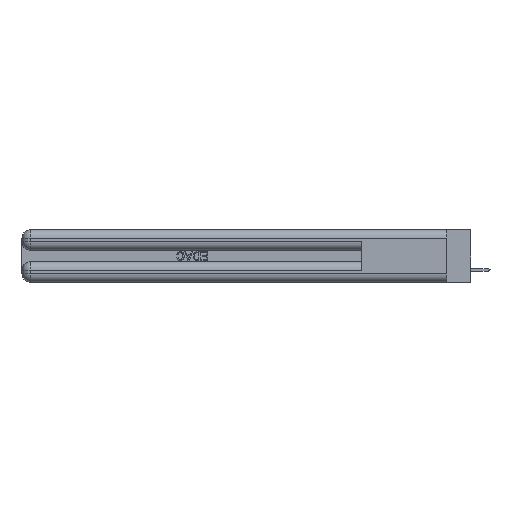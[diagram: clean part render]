
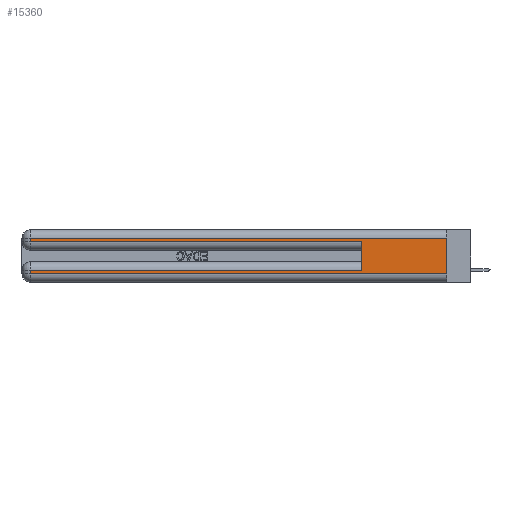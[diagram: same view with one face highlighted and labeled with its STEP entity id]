
A CAD part, left-side view. The second image highlights one B-rep face of the part: STEP entity #15360.
In plain terms, the highlighted planar face has unit normal (-1, 0, 0).
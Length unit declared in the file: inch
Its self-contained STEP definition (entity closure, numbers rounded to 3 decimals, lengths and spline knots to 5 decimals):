
#1582 = CARTESIAN_POINT ( 'NONE',  ( 0., 0.6, 0.285 ) ) ;
#2096 = CARTESIAN_POINT ( 'NONE',  ( 0., 2.94, 0.37 ) ) ;
#4617 = DIRECTION ( 'NONE',  ( 0., 1., 0. ) ) ;
#4679 = LINE ( 'NONE', #52619, #6367 ) ;
#5999 = ORIENTED_EDGE ( 'NONE', *, *, #34474, .T. ) ;
#6293 = VECTOR ( 'NONE', #22953, 39.37008 ) ;
#6367 = VECTOR ( 'NONE', #24795, 39.37008 ) ;
#7315 = LINE ( 'NONE', #24881, #41781 ) ;
#9867 = EDGE_CURVE ( 'NONE', #53524, #52220, #13985, .T. ) ;
#9911 = VERTEX_POINT ( 'NONE', #38701 ) ;
#11343 = ORIENTED_EDGE ( 'NONE', *, *, #21240, .T. ) ;
#13246 = ORIENTED_EDGE ( 'NONE', *, *, #28606, .F. ) ;
#13438 = FACE_OUTER_BOUND ( 'NONE', #19510, .T. ) ;
#13985 = LINE ( 'NONE', #18338, #6293 ) ;
#14717 = CARTESIAN_POINT ( 'NONE',  ( 0., 0., 0.37 ) ) ;
#14865 = VECTOR ( 'NONE', #4617, 39.37008 ) ;
#15360 = ADVANCED_FACE ( 'NONE', ( #13438 ), #34341, .F. ) ;
#17070 = ORIENTED_EDGE ( 'NONE', *, *, #25640, .T. ) ;
#17555 = ORIENTED_EDGE ( 'NONE', *, *, #9867, .T. ) ;
#17757 = CARTESIAN_POINT ( 'NONE',  ( 0., 2.94, 0.06 ) ) ;
#17925 = CARTESIAN_POINT ( 'NONE',  ( 0., 0., 0.31 ) ) ;
#18238 = VERTEX_POINT ( 'NONE', #35197 ) ;
#18338 = CARTESIAN_POINT ( 'NONE',  ( 0., 2.94, 0.37 ) ) ;
#19503 = CARTESIAN_POINT ( 'NONE',  ( 0., 2.94, 0.31 ) ) ;
#19510 = EDGE_LOOP ( 'NONE', ( #13246, #17070, #52996, #36879, #20248, #11343, #17555, #5999 ) ) ;
#20248 = ORIENTED_EDGE ( 'NONE', *, *, #52479, .F. ) ;
#21240 = EDGE_CURVE ( 'NONE', #18238, #53524, #4679, .T. ) ;
#22718 = LINE ( 'NONE', #2096, #28670 ) ;
#22953 = DIRECTION ( 'NONE',  ( 0., 0., -1. ) ) ;
#23076 = CARTESIAN_POINT ( 'NONE',  ( 0., 0., 0.06 ) ) ;
#24795 = DIRECTION ( 'NONE',  ( 0., 1., 0. ) ) ;
#24881 = CARTESIAN_POINT ( 'NONE',  ( 0., 0., 0.37 ) ) ;
#25640 = EDGE_CURVE ( 'NONE', #30573, #50424, #33668, .T. ) ;
#27232 = VERTEX_POINT ( 'NONE', #1582 ) ;
#27782 = DIRECTION ( 'NONE',  ( 0., 0., 1. ) ) ;
#27937 = LINE ( 'NONE', #23076, #38654 ) ;
#28046 = LINE ( 'NONE', #28839, #50780 ) ;
#28440 = CARTESIAN_POINT ( 'NONE',  ( 0., 2.94, 0.085 ) ) ;
#28606 = EDGE_CURVE ( 'NONE', #30573, #9911, #7315, .T. ) ;
#28670 = VECTOR ( 'NONE', #51251, 39.37008 ) ;
#28839 = CARTESIAN_POINT ( 'NONE',  ( 0., 0.6, 0.145 ) ) ;
#29768 = VECTOR ( 'NONE', #53421, 39.37008 ) ;
#30091 = EDGE_CURVE ( 'NONE', #37334, #27232, #32470, .T. ) ;
#30394 = CARTESIAN_POINT ( 'NONE',  ( 0., 0., 0.31 ) ) ;
#30573 = VERTEX_POINT ( 'NONE', #17925 ) ;
#32470 = LINE ( 'NONE', #41150, #29768 ) ;
#32953 = AXIS2_PLACEMENT_3D ( 'NONE', #14717, #38137, #48127 ) ;
#33668 = LINE ( 'NONE', #30394, #14865 ) ;
#34341 = PLANE ( 'NONE',  #32953 ) ;
#34474 = EDGE_CURVE ( 'NONE', #52220, #9911, #27937, .T. ) ;
#35197 = CARTESIAN_POINT ( 'NONE',  ( 0., 0.6, 0.085 ) ) ;
#36879 = ORIENTED_EDGE ( 'NONE', *, *, #30091, .T. ) ;
#37334 = VERTEX_POINT ( 'NONE', #41822 ) ;
#38137 = DIRECTION ( 'NONE',  ( 1., 0., 0. ) ) ;
#38654 = VECTOR ( 'NONE', #39628, 39.37008 ) ;
#38701 = CARTESIAN_POINT ( 'NONE',  ( 0., 0., 0.06 ) ) ;
#39628 = DIRECTION ( 'NONE',  ( 0., -1., 0. ) ) ;
#40443 = DIRECTION ( 'NONE',  ( 0., 0., -1. ) ) ;
#41150 = CARTESIAN_POINT ( 'NONE',  ( 0., 0., 0.285 ) ) ;
#41781 = VECTOR ( 'NONE', #40443, 39.37008 ) ;
#41822 = CARTESIAN_POINT ( 'NONE',  ( 0., 2.94, 0.285 ) ) ;
#45332 = EDGE_CURVE ( 'NONE', #50424, #37334, #22718, .T. ) ;
#48127 = DIRECTION ( 'NONE',  ( 0., 0., -1. ) ) ;
#50424 = VERTEX_POINT ( 'NONE', #19503 ) ;
#50780 = VECTOR ( 'NONE', #27782, 39.37008 ) ;
#51251 = DIRECTION ( 'NONE',  ( 0., 0., -1. ) ) ;
#52220 = VERTEX_POINT ( 'NONE', #17757 ) ;
#52479 = EDGE_CURVE ( 'NONE', #18238, #27232, #28046, .T. ) ;
#52619 = CARTESIAN_POINT ( 'NONE',  ( 0., 0., 0.085 ) ) ;
#52996 = ORIENTED_EDGE ( 'NONE', *, *, #45332, .T. ) ;
#53421 = DIRECTION ( 'NONE',  ( 0., -1., 0. ) ) ;
#53524 = VERTEX_POINT ( 'NONE', #28440 ) ;
